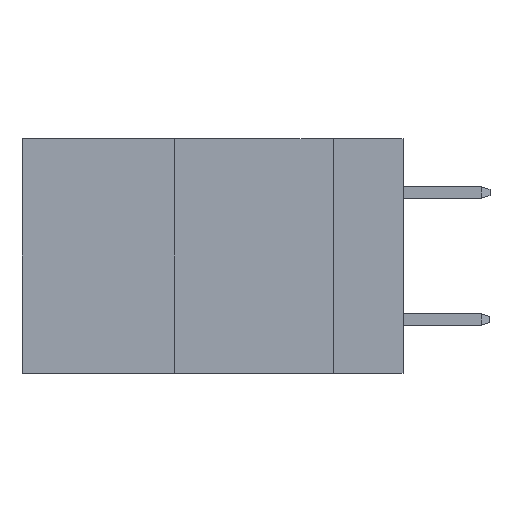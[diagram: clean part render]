
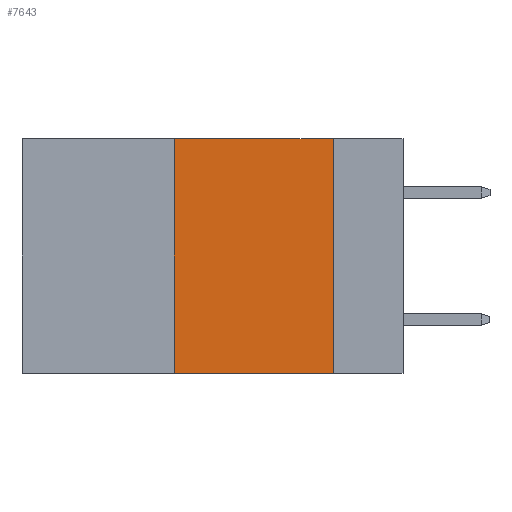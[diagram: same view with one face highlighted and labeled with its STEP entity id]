
A CAD part, left-side view. The second image highlights one B-rep face of the part: STEP entity #7643.
In plain terms, the highlighted planar face has unit normal (-1, 0, 0).
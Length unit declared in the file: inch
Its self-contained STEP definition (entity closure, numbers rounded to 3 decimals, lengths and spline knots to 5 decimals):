
#407 = CARTESIAN_POINT ( 'NONE',  ( 0., 0.6, 0. ) ) ;
#856 = VERTEX_POINT ( 'NONE', #5760 ) ;
#1176 = ORIENTED_EDGE ( 'NONE', *, *, #1291, .T. ) ;
#1291 = EDGE_CURVE ( 'NONE', #856, #7921, #4779, .T. ) ;
#1403 = CARTESIAN_POINT ( 'NONE',  ( 0., 0.6, 0. ) ) ;
#1519 = DIRECTION ( 'NONE',  ( 1., 0., 0. ) ) ;
#1573 = DIRECTION ( 'NONE',  ( 0., 0., -1. ) ) ;
#2227 = VECTOR ( 'NONE', #5815, 39.37008 ) ;
#3075 = CARTESIAN_POINT ( 'NONE',  ( 0., 0.11, 0. ) ) ;
#3245 = FACE_OUTER_BOUND ( 'NONE', #9409, .T. ) ;
#4257 = EDGE_CURVE ( 'NONE', #856, #7749, #10345, .T. ) ;
#4779 = LINE ( 'NONE', #7448, #2227 ) ;
#5129 = DIRECTION ( 'NONE',  ( 0., 0., 1. ) ) ;
#5147 = ORIENTED_EDGE ( 'NONE', *, *, #4257, .F. ) ;
#5182 = LINE ( 'NONE', #10394, #7389 ) ;
#5257 = ORIENTED_EDGE ( 'NONE', *, *, #9549, .F. ) ;
#5642 = DIRECTION ( 'NONE',  ( 0., -1., 0. ) ) ;
#5760 = CARTESIAN_POINT ( 'NONE',  ( 0., 0.36, -0.37 ) ) ;
#5815 = DIRECTION ( 'NONE',  ( 0., -1., 0. ) ) ;
#6282 = VERTEX_POINT ( 'NONE', #3075 ) ;
#6427 = VECTOR ( 'NONE', #5642, 39.37008 ) ;
#7106 = DIRECTION ( 'NONE',  ( 0., 0., -1. ) ) ;
#7389 = VECTOR ( 'NONE', #7106, 39.37008 ) ;
#7402 = CARTESIAN_POINT ( 'NONE',  ( 0., 0.11, -0.37 ) ) ;
#7448 = CARTESIAN_POINT ( 'NONE',  ( 0., 0.6, -0.37 ) ) ;
#7479 = ORIENTED_EDGE ( 'NONE', *, *, #7882, .F. ) ;
#7643 = ADVANCED_FACE ( 'NONE', ( #3245 ), #8449, .F. ) ;
#7689 = CARTESIAN_POINT ( 'NONE',  ( 0., 0.36, 0. ) ) ;
#7749 = VERTEX_POINT ( 'NONE', #9673 ) ;
#7882 = EDGE_CURVE ( 'NONE', #7749, #6282, #10665, .T. ) ;
#7921 = VERTEX_POINT ( 'NONE', #7402 ) ;
#7932 = AXIS2_PLACEMENT_3D ( 'NONE', #1403, #1519, #1573 ) ;
#8449 = PLANE ( 'NONE',  #7932 ) ;
#9409 = EDGE_LOOP ( 'NONE', ( #5257, #7479, #5147, #1176 ) ) ;
#9526 = VECTOR ( 'NONE', #5129, 39.37008 ) ;
#9549 = EDGE_CURVE ( 'NONE', #6282, #7921, #5182, .T. ) ;
#9673 = CARTESIAN_POINT ( 'NONE',  ( 0., 0.36, 0. ) ) ;
#10345 = LINE ( 'NONE', #7689, #9526 ) ;
#10394 = CARTESIAN_POINT ( 'NONE',  ( 0., 0.11, 0. ) ) ;
#10665 = LINE ( 'NONE', #407, #6427 ) ;
